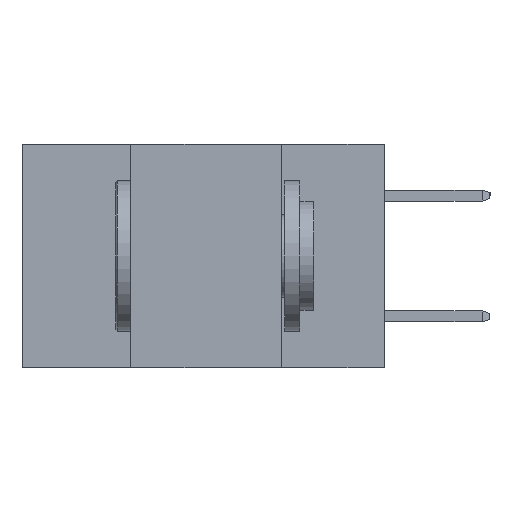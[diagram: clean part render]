
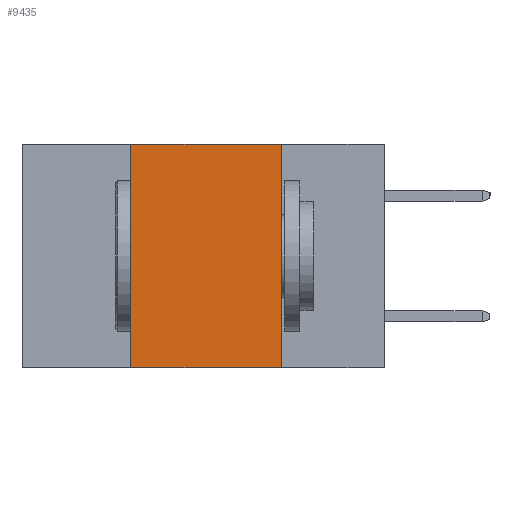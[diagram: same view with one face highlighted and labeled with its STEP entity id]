
A CAD part, left-side view. The second image highlights one B-rep face of the part: STEP entity #9435.
In plain terms, the highlighted planar face has unit normal (-1, 0, 0).
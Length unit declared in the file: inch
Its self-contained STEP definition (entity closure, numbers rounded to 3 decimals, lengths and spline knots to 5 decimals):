
#168 = LINE ( 'NONE', #2557, #12112 ) ;
#1135 = EDGE_CURVE ( 'NONE', #9705, #4624, #20057, .T. ) ;
#2063 = FACE_OUTER_BOUND ( 'NONE', #17891, .T. ) ;
#2557 = CARTESIAN_POINT ( 'NONE',  ( 0., 0.42, -0.37 ) ) ;
#3391 = VECTOR ( 'NONE', #20314, 39.37008 ) ;
#3797 = DIRECTION ( 'NONE',  ( 0., 0., -1. ) ) ;
#4624 = VERTEX_POINT ( 'NONE', #7431 ) ;
#5914 = CARTESIAN_POINT ( 'NONE',  ( 0., 0.6, 0. ) ) ;
#5983 = ORIENTED_EDGE ( 'NONE', *, *, #6651, .T. ) ;
#6651 = EDGE_CURVE ( 'NONE', #11818, #4624, #7305, .T. ) ;
#7182 = CARTESIAN_POINT ( 'NONE',  ( 0., 0.17, -0.37 ) ) ;
#7305 = LINE ( 'NONE', #11673, #3391 ) ;
#7431 = CARTESIAN_POINT ( 'NONE',  ( 0., 0.17, -0.37 ) ) ;
#8516 = ORIENTED_EDGE ( 'NONE', *, *, #1135, .F. ) ;
#9435 = ADVANCED_FACE ( 'NONE', ( #2063 ), #17227, .F. ) ;
#9705 = VERTEX_POINT ( 'NONE', #24814 ) ;
#10544 = EDGE_CURVE ( 'NONE', #11818, #15204, #168, .T. ) ;
#11286 = CARTESIAN_POINT ( 'NONE',  ( 0., 0.42, 0. ) ) ;
#11558 = DIRECTION ( 'NONE',  ( 0., 0., -1. ) ) ;
#11673 = CARTESIAN_POINT ( 'NONE',  ( 0., 0.6, -0.37 ) ) ;
#11712 = EDGE_CURVE ( 'NONE', #15204, #9705, #17165, .T. ) ;
#11818 = VERTEX_POINT ( 'NONE', #26167 ) ;
#12112 = VECTOR ( 'NONE', #17574, 39.37008 ) ;
#13456 = ORIENTED_EDGE ( 'NONE', *, *, #10544, .F. ) ;
#15204 = VERTEX_POINT ( 'NONE', #11286 ) ;
#16864 = ORIENTED_EDGE ( 'NONE', *, *, #11712, .F. ) ;
#17165 = LINE ( 'NONE', #21250, #23005 ) ;
#17227 = PLANE ( 'NONE',  #24257 ) ;
#17574 = DIRECTION ( 'NONE',  ( 0., 0., 1. ) ) ;
#17891 = EDGE_LOOP ( 'NONE', ( #8516, #16864, #13456, #5983 ) ) ;
#19276 = DIRECTION ( 'NONE',  ( 0., -1., 0. ) ) ;
#20057 = LINE ( 'NONE', #7182, #26186 ) ;
#20314 = DIRECTION ( 'NONE',  ( 0., -1., 0. ) ) ;
#21250 = CARTESIAN_POINT ( 'NONE',  ( 0., 0.6, 0. ) ) ;
#23005 = VECTOR ( 'NONE', #19276, 39.37008 ) ;
#24257 = AXIS2_PLACEMENT_3D ( 'NONE', #5914, #27801, #3797 ) ;
#24814 = CARTESIAN_POINT ( 'NONE',  ( 0., 0.17, 0. ) ) ;
#26167 = CARTESIAN_POINT ( 'NONE',  ( 0., 0.42, -0.37 ) ) ;
#26186 = VECTOR ( 'NONE', #11558, 39.37008 ) ;
#27801 = DIRECTION ( 'NONE',  ( 1., 0., 0. ) ) ;
